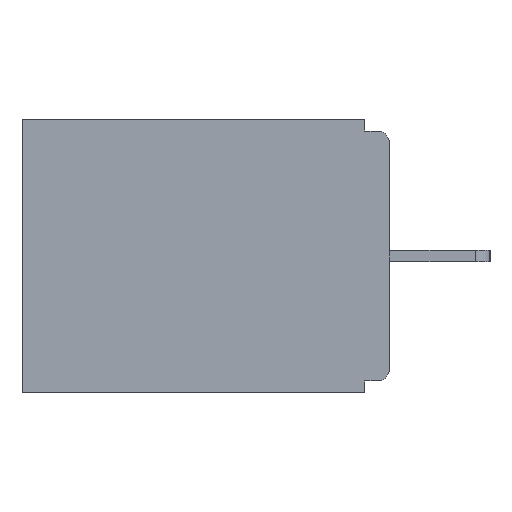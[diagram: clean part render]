
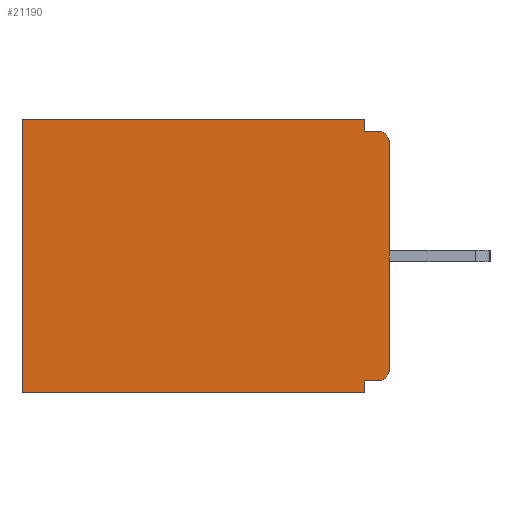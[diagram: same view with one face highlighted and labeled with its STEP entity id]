
A CAD part, left-side view. The second image highlights one B-rep face of the part: STEP entity #21190.
In plain terms, the highlighted planar face has unit normal (-1, 0, 0).
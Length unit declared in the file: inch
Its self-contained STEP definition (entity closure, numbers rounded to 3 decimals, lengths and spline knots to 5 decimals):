
#358 = DIRECTION ( 'NONE',  ( 0., 0., -1. ) ) ;
#431 = DIRECTION ( 'NONE',  ( -1., 0., 0. ) ) ;
#620 = EDGE_CURVE ( 'NONE', #2463, #21706, #9098, .T. ) ;
#935 = DIRECTION ( 'NONE',  ( -1., 0., 0. ) ) ;
#1114 = ORIENTED_EDGE ( 'NONE', *, *, #16034, .F. ) ;
#1393 = CARTESIAN_POINT ( 'NONE',  ( 0.298, 0.46, 0. ) ) ;
#1732 = ORIENTED_EDGE ( 'NONE', *, *, #16814, .F. ) ;
#2209 = DIRECTION ( 'NONE',  ( 0., 0., -1. ) ) ;
#2463 = VERTEX_POINT ( 'NONE', #22198 ) ;
#2773 = AXIS2_PLACEMENT_3D ( 'NONE', #18431, #935, #4906 ) ;
#3268 = CARTESIAN_POINT ( 'NONE',  ( 0.298, 0.46, -0.343 ) ) ;
#3365 = CARTESIAN_POINT ( 'NONE',  ( 0.298, 0., 0. ) ) ;
#3596 = DIRECTION ( 'NONE',  ( 1., 0., 0. ) ) ;
#3764 = DIRECTION ( 'NONE',  ( 0., 1., 0. ) ) ;
#3811 = LINE ( 'NONE', #13628, #24208 ) ;
#3893 = VECTOR ( 'NONE', #12835, 39.37008 ) ;
#4163 = EDGE_CURVE ( 'NONE', #6804, #16140, #13979, .T. ) ;
#4383 = VERTEX_POINT ( 'NONE', #3268 ) ;
#4566 = EDGE_CURVE ( 'NONE', #25046, #12686, #19835, .T. ) ;
#4906 = DIRECTION ( 'NONE',  ( 0., 0., -1. ) ) ;
#5416 = EDGE_CURVE ( 'NONE', #2463, #10694, #16154, .T. ) ;
#5507 = CARTESIAN_POINT ( 'NONE',  ( 0.298, 0., 0. ) ) ;
#5683 = DIRECTION ( 'NONE',  ( 0., -1., 0. ) ) ;
#6046 = CARTESIAN_POINT ( 'NONE',  ( 0.298, 0., -0.015 ) ) ;
#6077 = VECTOR ( 'NONE', #3764, 39.37008 ) ;
#6331 = DIRECTION ( 'NONE',  ( 0., 1., 0. ) ) ;
#6397 = CARTESIAN_POINT ( 'NONE',  ( 0.298, 0., -0.03 ) ) ;
#6804 = VERTEX_POINT ( 'NONE', #9251 ) ;
#6837 = EDGE_CURVE ( 'NONE', #23494, #4383, #14993, .T. ) ;
#7118 = LINE ( 'NONE', #11167, #3893 ) ;
#7560 = LINE ( 'NONE', #5507, #17328 ) ;
#8479 = ORIENTED_EDGE ( 'NONE', *, *, #620, .T. ) ;
#8535 = EDGE_CURVE ( 'NONE', #6804, #19610, #10521, .T. ) ;
#8652 = CARTESIAN_POINT ( 'NONE',  ( 0.298, 0.031, -0.343 ) ) ;
#9098 = LINE ( 'NONE', #3365, #24128 ) ;
#9251 = CARTESIAN_POINT ( 'NONE',  ( 0.298, 0.015, -0.328 ) ) ;
#9401 = ORIENTED_EDGE ( 'NONE', *, *, #4566, .T. ) ;
#9600 = CARTESIAN_POINT ( 'NONE',  ( 0.298, 0.015, -0.015 ) ) ;
#10494 = VECTOR ( 'NONE', #17817, 39.37008 ) ;
#10521 = CIRCLE ( 'NONE', #2773, 0.015 ) ;
#10694 = VERTEX_POINT ( 'NONE', #18826 ) ;
#11167 = CARTESIAN_POINT ( 'NONE',  ( 0.298, 0.031, -0.343 ) ) ;
#11381 = CARTESIAN_POINT ( 'NONE',  ( 0.298, 0., 0. ) ) ;
#11788 = EDGE_LOOP ( 'NONE', ( #9401, #14490, #18576, #8479, #17942, #24331, #1732, #24196, #14914, #1114 ) ) ;
#12209 = CARTESIAN_POINT ( 'NONE',  ( 0.298, 0., -0.328 ) ) ;
#12686 = VERTEX_POINT ( 'NONE', #9600 ) ;
#12790 = DIRECTION ( 'NONE',  ( 0., 1., 0. ) ) ;
#12835 = DIRECTION ( 'NONE',  ( 0., 0., -1. ) ) ;
#12900 = DIRECTION ( 'NONE',  ( 0., 0., -1. ) ) ;
#13579 = LINE ( 'NONE', #6046, #13865 ) ;
#13628 = CARTESIAN_POINT ( 'NONE',  ( 0.298, 0.46, 0. ) ) ;
#13865 = VECTOR ( 'NONE', #5683, 39.37008 ) ;
#13979 = LINE ( 'NONE', #12209, #18606 ) ;
#14490 = ORIENTED_EDGE ( 'NONE', *, *, #24445, .F. ) ;
#14820 = PLANE ( 'NONE',  #19907 ) ;
#14914 = ORIENTED_EDGE ( 'NONE', *, *, #8535, .T. ) ;
#14993 = LINE ( 'NONE', #17400, #6077 ) ;
#15736 = EDGE_CURVE ( 'NONE', #21706, #4383, #3811, .T. ) ;
#15738 = CARTESIAN_POINT ( 'NONE',  ( 0.298, 0.015, -0.03 ) ) ;
#16034 = EDGE_CURVE ( 'NONE', #25046, #19610, #7560, .T. ) ;
#16140 = VERTEX_POINT ( 'NONE', #23223 ) ;
#16154 = LINE ( 'NONE', #8652, #10494 ) ;
#16746 = FACE_OUTER_BOUND ( 'NONE', #11788, .T. ) ;
#16814 = EDGE_CURVE ( 'NONE', #16140, #23494, #7118, .T. ) ;
#17328 = VECTOR ( 'NONE', #20927, 39.37008 ) ;
#17400 = CARTESIAN_POINT ( 'NONE',  ( 0.298, 0., -0.343 ) ) ;
#17793 = AXIS2_PLACEMENT_3D ( 'NONE', #15738, #431, #2209 ) ;
#17817 = DIRECTION ( 'NONE',  ( 0., 0., -1. ) ) ;
#17942 = ORIENTED_EDGE ( 'NONE', *, *, #15736, .T. ) ;
#18431 = CARTESIAN_POINT ( 'NONE',  ( 0.298, 0.015, -0.313 ) ) ;
#18576 = ORIENTED_EDGE ( 'NONE', *, *, #5416, .F. ) ;
#18606 = VECTOR ( 'NONE', #6331, 39.37008 ) ;
#18826 = CARTESIAN_POINT ( 'NONE',  ( 0.298, 0.031, -0.015 ) ) ;
#19610 = VERTEX_POINT ( 'NONE', #19672 ) ;
#19672 = CARTESIAN_POINT ( 'NONE',  ( 0.298, 0., -0.313 ) ) ;
#19835 = CIRCLE ( 'NONE', #17793, 0.015 ) ;
#19907 = AXIS2_PLACEMENT_3D ( 'NONE', #11381, #3596, #12900 ) ;
#20927 = DIRECTION ( 'NONE',  ( 0., 0., -1. ) ) ;
#21190 = ADVANCED_FACE ( 'NONE', ( #16746 ), #14820, .F. ) ;
#21706 = VERTEX_POINT ( 'NONE', #1393 ) ;
#21757 = CARTESIAN_POINT ( 'NONE',  ( 0.298, 0.031, -0.343 ) ) ;
#22198 = CARTESIAN_POINT ( 'NONE',  ( 0.298, 0.031, 0. ) ) ;
#23223 = CARTESIAN_POINT ( 'NONE',  ( 0.298, 0.031, -0.328 ) ) ;
#23494 = VERTEX_POINT ( 'NONE', #21757 ) ;
#24128 = VECTOR ( 'NONE', #12790, 39.37008 ) ;
#24196 = ORIENTED_EDGE ( 'NONE', *, *, #4163, .F. ) ;
#24208 = VECTOR ( 'NONE', #358, 39.37008 ) ;
#24331 = ORIENTED_EDGE ( 'NONE', *, *, #6837, .F. ) ;
#24445 = EDGE_CURVE ( 'NONE', #10694, #12686, #13579, .T. ) ;
#25046 = VERTEX_POINT ( 'NONE', #6397 ) ;
